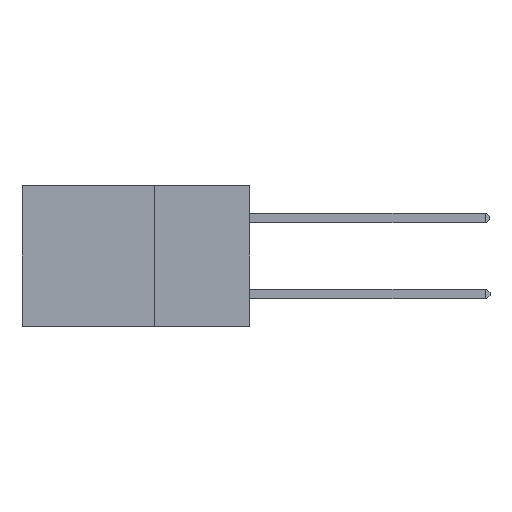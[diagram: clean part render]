
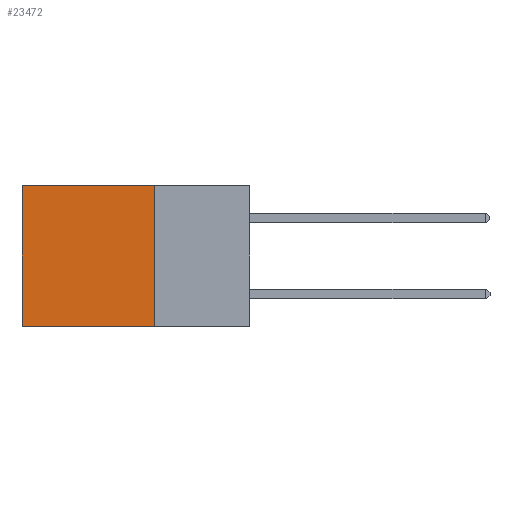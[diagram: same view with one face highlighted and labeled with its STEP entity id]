
A CAD part, left-side view. The second image highlights one B-rep face of the part: STEP entity #23472.
In plain terms, the highlighted planar face has unit normal (-1, 0, 0).
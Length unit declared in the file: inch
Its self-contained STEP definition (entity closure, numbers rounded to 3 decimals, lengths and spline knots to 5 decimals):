
#575 = VECTOR ( 'NONE', #17987, 39.37008 ) ;
#595 = DIRECTION ( 'NONE',  ( 1., 0., 0. ) ) ;
#694 = DIRECTION ( 'NONE',  ( 0., 0., -1. ) ) ;
#1419 = DIRECTION ( 'NONE',  ( 0., 1., 0. ) ) ;
#2857 = EDGE_CURVE ( 'NONE', #8378, #21368, #5549, .T. ) ;
#3553 = EDGE_LOOP ( 'NONE', ( #18918, #13058, #11912, #14399 ) ) ;
#4084 = CARTESIAN_POINT ( 'NONE',  ( 0.2875, 0.6, 0. ) ) ;
#5549 = LINE ( 'NONE', #19687, #575 ) ;
#5922 = FACE_OUTER_BOUND ( 'NONE', #3553, .T. ) ;
#6154 = CARTESIAN_POINT ( 'NONE',  ( 0.2875, 0.25, 0. ) ) ;
#7891 = EDGE_CURVE ( 'NONE', #19230, #8378, #19519, .T. ) ;
#8378 = VERTEX_POINT ( 'NONE', #11739 ) ;
#8550 = DIRECTION ( 'NONE',  ( 0., 0., -1. ) ) ;
#9327 = EDGE_CURVE ( 'NONE', #19230, #14963, #14763, .T. ) ;
#9379 = CARTESIAN_POINT ( 'NONE',  ( 0.2875, 0.6, -0.37 ) ) ;
#9923 = VECTOR ( 'NONE', #1419, 39.37008 ) ;
#10476 = VECTOR ( 'NONE', #8550, 39.37008 ) ;
#10996 = LINE ( 'NONE', #11792, #20013 ) ;
#11017 = EDGE_CURVE ( 'NONE', #14963, #21368, #10996, .T. ) ;
#11739 = CARTESIAN_POINT ( 'NONE',  ( 0.2875, 0.25, -0.37 ) ) ;
#11792 = CARTESIAN_POINT ( 'NONE',  ( 0.2875, 0.6, 0. ) ) ;
#11912 = ORIENTED_EDGE ( 'NONE', *, *, #7891, .F. ) ;
#13058 = ORIENTED_EDGE ( 'NONE', *, *, #2857, .F. ) ;
#13546 = DIRECTION ( 'NONE',  ( 0., 0., -1. ) ) ;
#14399 = ORIENTED_EDGE ( 'NONE', *, *, #9327, .T. ) ;
#14763 = LINE ( 'NONE', #23239, #9923 ) ;
#14963 = VERTEX_POINT ( 'NONE', #4084 ) ;
#17230 = AXIS2_PLACEMENT_3D ( 'NONE', #6154, #595, #13546 ) ;
#17987 = DIRECTION ( 'NONE',  ( 0., 1., 0. ) ) ;
#18892 = PLANE ( 'NONE',  #17230 ) ;
#18918 = ORIENTED_EDGE ( 'NONE', *, *, #11017, .T. ) ;
#19230 = VERTEX_POINT ( 'NONE', #21153 ) ;
#19405 = CARTESIAN_POINT ( 'NONE',  ( 0.2875, 0.25, 0. ) ) ;
#19519 = LINE ( 'NONE', #19405, #10476 ) ;
#19687 = CARTESIAN_POINT ( 'NONE',  ( 0.2875, 0.25, -0.37 ) ) ;
#20013 = VECTOR ( 'NONE', #694, 39.37008 ) ;
#21153 = CARTESIAN_POINT ( 'NONE',  ( 0.2875, 0.25, 0. ) ) ;
#21368 = VERTEX_POINT ( 'NONE', #9379 ) ;
#23239 = CARTESIAN_POINT ( 'NONE',  ( 0.2875, 0.25, 0. ) ) ;
#23472 = ADVANCED_FACE ( 'NONE', ( #5922 ), #18892, .F. ) ;
